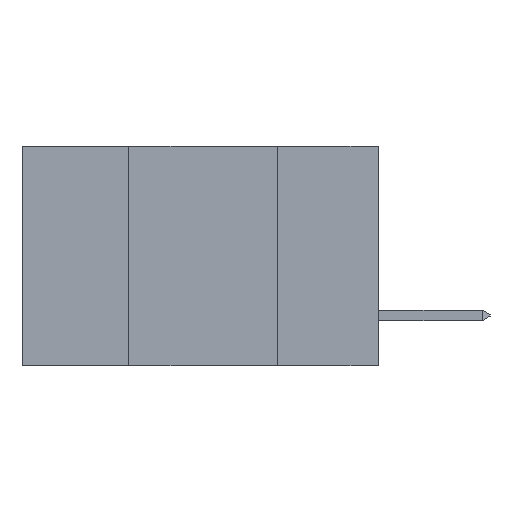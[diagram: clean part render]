
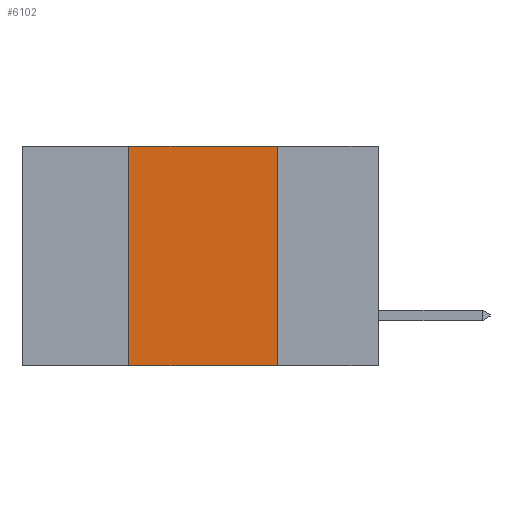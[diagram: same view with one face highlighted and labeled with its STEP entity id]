
A CAD part, left-side view. The second image highlights one B-rep face of the part: STEP entity #6102.
In plain terms, the highlighted planar face has unit normal (-1, 0, 0).
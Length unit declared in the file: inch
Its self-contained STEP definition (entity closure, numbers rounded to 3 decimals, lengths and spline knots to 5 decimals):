
#404 = AXIS2_PLACEMENT_3D ( 'NONE', #14521, #9716, #20625 ) ;
#2035 = CARTESIAN_POINT ( 'NONE',  ( 0., 0.17, 0. ) ) ;
#2351 = CARTESIAN_POINT ( 'NONE',  ( 0., 0.6, 0. ) ) ;
#2596 = LINE ( 'NONE', #6136, #15172 ) ;
#3854 = ORIENTED_EDGE ( 'NONE', *, *, #12173, .F. ) ;
#3973 = CARTESIAN_POINT ( 'NONE',  ( 0., 0.6, -0.37 ) ) ;
#4056 = DIRECTION ( 'NONE',  ( 0., -1., 0. ) ) ;
#4069 = ORIENTED_EDGE ( 'NONE', *, *, #11076, .F. ) ;
#4545 = EDGE_LOOP ( 'NONE', ( #3854, #4069, #5135, #5723 ) ) ;
#4880 = VERTEX_POINT ( 'NONE', #7820 ) ;
#5135 = ORIENTED_EDGE ( 'NONE', *, *, #9963, .F. ) ;
#5723 = ORIENTED_EDGE ( 'NONE', *, *, #7723, .T. ) ;
#6102 = ADVANCED_FACE ( 'NONE', ( #16461 ), #8019, .F. ) ;
#6136 = CARTESIAN_POINT ( 'NONE',  ( 0., 0.42, -0.37 ) ) ;
#7320 = DIRECTION ( 'NONE',  ( 0., -1., 0. ) ) ;
#7723 = EDGE_CURVE ( 'NONE', #4880, #11260, #15191, .T. ) ;
#7820 = CARTESIAN_POINT ( 'NONE',  ( 0., 0.42, -0.37 ) ) ;
#8019 = PLANE ( 'NONE',  #404 ) ;
#8259 = VERTEX_POINT ( 'NONE', #2035 ) ;
#9716 = DIRECTION ( 'NONE',  ( 1., 0., 0. ) ) ;
#9963 = EDGE_CURVE ( 'NONE', #4880, #12966, #2596, .T. ) ;
#10986 = VECTOR ( 'NONE', #7320, 39.37008 ) ;
#11076 = EDGE_CURVE ( 'NONE', #12966, #8259, #17573, .T. ) ;
#11260 = VERTEX_POINT ( 'NONE', #12811 ) ;
#12173 = EDGE_CURVE ( 'NONE', #8259, #11260, #17761, .T. ) ;
#12811 = CARTESIAN_POINT ( 'NONE',  ( 0., 0.17, -0.37 ) ) ;
#12966 = VERTEX_POINT ( 'NONE', #15540 ) ;
#12979 = VECTOR ( 'NONE', #4056, 39.37008 ) ;
#13646 = DIRECTION ( 'NONE',  ( 0., 0., -1. ) ) ;
#13712 = CARTESIAN_POINT ( 'NONE',  ( 0., 0.17, -0.37 ) ) ;
#14521 = CARTESIAN_POINT ( 'NONE',  ( 0., 0.6, 0. ) ) ;
#15172 = VECTOR ( 'NONE', #20421, 39.37008 ) ;
#15191 = LINE ( 'NONE', #3973, #10986 ) ;
#15540 = CARTESIAN_POINT ( 'NONE',  ( 0., 0.42, 0. ) ) ;
#16461 = FACE_OUTER_BOUND ( 'NONE', #4545, .T. ) ;
#17273 = VECTOR ( 'NONE', #13646, 39.37008 ) ;
#17573 = LINE ( 'NONE', #2351, #12979 ) ;
#17761 = LINE ( 'NONE', #13712, #17273 ) ;
#20421 = DIRECTION ( 'NONE',  ( 0., 0., 1. ) ) ;
#20625 = DIRECTION ( 'NONE',  ( 0., 0., -1. ) ) ;
